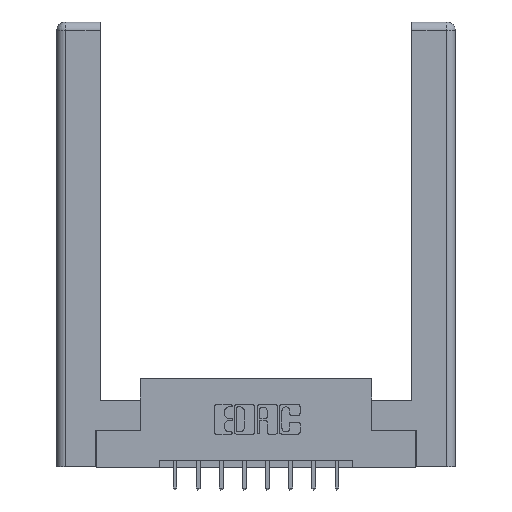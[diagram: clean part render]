
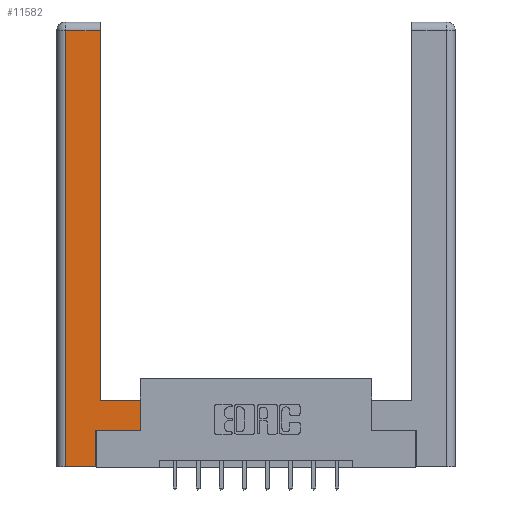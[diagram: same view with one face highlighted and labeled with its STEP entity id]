
A CAD part, top view. The second image highlights one B-rep face of the part: STEP entity #11582.
In plain terms, the highlighted planar face has unit normal (0, 0, 1).
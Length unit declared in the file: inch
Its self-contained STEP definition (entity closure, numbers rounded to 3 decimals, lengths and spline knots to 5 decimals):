
#104 = LINE ( 'NONE', #3274, #10044 ) ;
#163 = DIRECTION ( 'NONE',  ( -1., 0., 0. ) ) ;
#1509 = AXIS2_PLACEMENT_3D ( 'NONE', #6622, #12646, #6579 ) ;
#1552 = CARTESIAN_POINT ( 'NONE',  ( 0.565, 0.245, 0. ) ) ;
#1610 = EDGE_LOOP ( 'NONE', ( #4747, #9920, #2692, #9961, #12532, #2967, #7802, #9832 ) ) ;
#1870 = VERTEX_POINT ( 'NONE', #9646 ) ;
#1886 = LINE ( 'NONE', #9644, #3516 ) ;
#1922 = CARTESIAN_POINT ( 'NONE',  ( 0.565, 0.45, 0. ) ) ;
#1961 = LINE ( 'NONE', #2042, #12214 ) ;
#1995 = DIRECTION ( 'NONE',  ( 0., 1., 0. ) ) ;
#2042 = CARTESIAN_POINT ( 'NONE',  ( 0.295, 3., 0. ) ) ;
#2253 = CARTESIAN_POINT ( 'NONE',  ( 0.265, 0., 0. ) ) ;
#2257 = DIRECTION ( 'NONE',  ( 1., 0., 0. ) ) ;
#2363 = VERTEX_POINT ( 'NONE', #7580 ) ;
#2692 = ORIENTED_EDGE ( 'NONE', *, *, #9073, .T. ) ;
#2967 = ORIENTED_EDGE ( 'NONE', *, *, #3092, .T. ) ;
#3092 = EDGE_CURVE ( 'NONE', #7752, #11074, #7335, .T. ) ;
#3157 = VERTEX_POINT ( 'NONE', #8556 ) ;
#3274 = CARTESIAN_POINT ( 'NONE',  ( 0.295, 0.45, 0. ) ) ;
#3516 = VECTOR ( 'NONE', #11654, 39.37008 ) ;
#4590 = CARTESIAN_POINT ( 'NONE',  ( 0.0615, 2.94, 0. ) ) ;
#4676 = LINE ( 'NONE', #1922, #5299 ) ;
#4747 = ORIENTED_EDGE ( 'NONE', *, *, #5557, .T. ) ;
#4958 = VERTEX_POINT ( 'NONE', #5531 ) ;
#5281 = EDGE_CURVE ( 'NONE', #12328, #2363, #5843, .T. ) ;
#5299 = VECTOR ( 'NONE', #12176, 39.37008 ) ;
#5531 = CARTESIAN_POINT ( 'NONE',  ( 0.295, 2.94, 0. ) ) ;
#5557 = EDGE_CURVE ( 'NONE', #1870, #4958, #1961, .T. ) ;
#5597 = CARTESIAN_POINT ( 'NONE',  ( 0.0615, 0., 0. ) ) ;
#5843 = LINE ( 'NONE', #2253, #13180 ) ;
#6427 = VECTOR ( 'NONE', #7012, 39.37008 ) ;
#6579 = DIRECTION ( 'NONE',  ( -1., 0., 0. ) ) ;
#6622 = CARTESIAN_POINT ( 'NONE',  ( 0., 0., 0. ) ) ;
#7000 = FACE_OUTER_BOUND ( 'NONE', #1610, .T. ) ;
#7012 = DIRECTION ( 'NONE',  ( 0., -1., 0. ) ) ;
#7034 = VECTOR ( 'NONE', #2257, 39.37008 ) ;
#7135 = VERTEX_POINT ( 'NONE', #7820 ) ;
#7303 = LINE ( 'NONE', #4590, #13045 ) ;
#7335 = LINE ( 'NONE', #9356, #7034 ) ;
#7580 = CARTESIAN_POINT ( 'NONE',  ( 0.265, 0., 0. ) ) ;
#7752 = VERTEX_POINT ( 'NONE', #8179 ) ;
#7802 = ORIENTED_EDGE ( 'NONE', *, *, #8860, .T. ) ;
#7820 = CARTESIAN_POINT ( 'NONE',  ( 0.0615, 2.94, 0. ) ) ;
#8008 = CARTESIAN_POINT ( 'NONE',  ( 0.0615, 0., 0. ) ) ;
#8149 = EDGE_CURVE ( 'NONE', #2363, #7752, #1886, .T. ) ;
#8179 = CARTESIAN_POINT ( 'NONE',  ( 0.265, 0.245, 0. ) ) ;
#8509 = DIRECTION ( 'NONE',  ( 1., 0., 0. ) ) ;
#8556 = CARTESIAN_POINT ( 'NONE',  ( 0.565, 0.45, 0. ) ) ;
#8584 = DIRECTION ( 'NONE',  ( -1., 0., 0. ) ) ;
#8860 = EDGE_CURVE ( 'NONE', #11074, #3157, #4676, .T. ) ;
#9073 = EDGE_CURVE ( 'NONE', #7135, #12328, #9431, .T. ) ;
#9356 = CARTESIAN_POINT ( 'NONE',  ( 0.565, 0.245, 0. ) ) ;
#9431 = LINE ( 'NONE', #8008, #6427 ) ;
#9644 = CARTESIAN_POINT ( 'NONE',  ( 0.265, 0.245, 0. ) ) ;
#9646 = CARTESIAN_POINT ( 'NONE',  ( 0.295, 0.45, 0. ) ) ;
#9832 = ORIENTED_EDGE ( 'NONE', *, *, #10329, .T. ) ;
#9920 = ORIENTED_EDGE ( 'NONE', *, *, #11634, .T. ) ;
#9961 = ORIENTED_EDGE ( 'NONE', *, *, #5281, .T. ) ;
#10044 = VECTOR ( 'NONE', #163, 39.37008 ) ;
#10329 = EDGE_CURVE ( 'NONE', #3157, #1870, #104, .T. ) ;
#11074 = VERTEX_POINT ( 'NONE', #1552 ) ;
#11582 = ADVANCED_FACE ( 'NONE', ( #7000 ), #11625, .F. ) ;
#11625 = PLANE ( 'NONE',  #1509 ) ;
#11634 = EDGE_CURVE ( 'NONE', #4958, #7135, #7303, .T. ) ;
#11654 = DIRECTION ( 'NONE',  ( 0., 1., 0. ) ) ;
#12176 = DIRECTION ( 'NONE',  ( 0., 1., 0. ) ) ;
#12214 = VECTOR ( 'NONE', #1995, 39.37008 ) ;
#12328 = VERTEX_POINT ( 'NONE', #5597 ) ;
#12532 = ORIENTED_EDGE ( 'NONE', *, *, #8149, .T. ) ;
#12646 = DIRECTION ( 'NONE',  ( 0., 0., -1. ) ) ;
#13045 = VECTOR ( 'NONE', #8584, 39.37008 ) ;
#13180 = VECTOR ( 'NONE', #8509, 39.37008 ) ;
